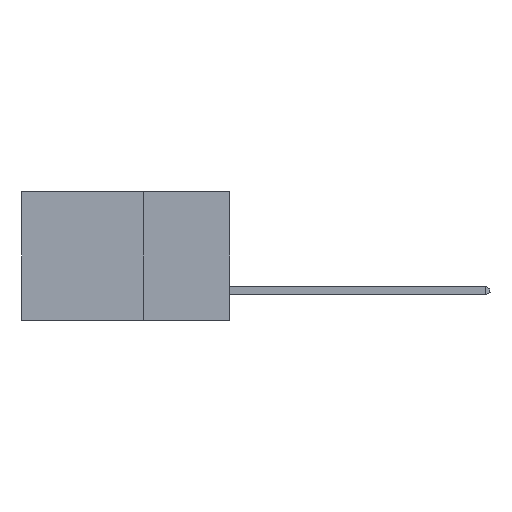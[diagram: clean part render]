
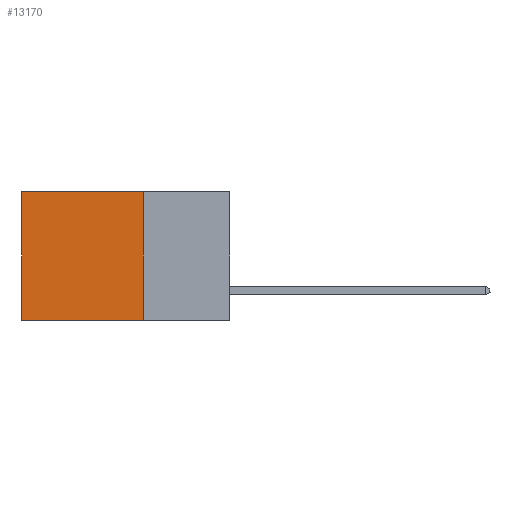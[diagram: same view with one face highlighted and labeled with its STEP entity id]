
A CAD part, left-side view. The second image highlights one B-rep face of the part: STEP entity #13170.
In plain terms, the highlighted planar face has unit normal (-1, 0, 0).
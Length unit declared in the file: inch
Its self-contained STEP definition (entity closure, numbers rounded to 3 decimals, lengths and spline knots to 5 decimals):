
#212 = LINE ( 'NONE', #4248, #2225 ) ;
#361 = DIRECTION ( 'NONE',  ( 1., 0., 0. ) ) ;
#650 = LINE ( 'NONE', #12073, #17280 ) ;
#757 = LINE ( 'NONE', #10620, #15401 ) ;
#853 = VERTEX_POINT ( 'NONE', #14147 ) ;
#2225 = VECTOR ( 'NONE', #9693, 39.37008 ) ;
#2422 = EDGE_CURVE ( 'NONE', #6569, #853, #212, .T. ) ;
#2776 = EDGE_CURVE ( 'NONE', #10429, #11926, #650, .T. ) ;
#3366 = ORIENTED_EDGE ( 'NONE', *, *, #5352, .T. ) ;
#4248 = CARTESIAN_POINT ( 'NONE',  ( 0.298, 0.25, 0. ) ) ;
#4781 = PLANE ( 'NONE',  #13228 ) ;
#5352 = EDGE_CURVE ( 'NONE', #853, #11926, #757, .T. ) ;
#5887 = DIRECTION ( 'NONE',  ( 0., 0., -1. ) ) ;
#6569 = VERTEX_POINT ( 'NONE', #12617 ) ;
#7108 = FACE_OUTER_BOUND ( 'NONE', #10901, .T. ) ;
#7660 = CARTESIAN_POINT ( 'NONE',  ( 0.298, 0.25, -0.37 ) ) ;
#9371 = DIRECTION ( 'NONE',  ( 0., 1., 0. ) ) ;
#9376 = ORIENTED_EDGE ( 'NONE', *, *, #2776, .F. ) ;
#9652 = ORIENTED_EDGE ( 'NONE', *, *, #2422, .T. ) ;
#9693 = DIRECTION ( 'NONE',  ( 0., 1., 0. ) ) ;
#10429 = VERTEX_POINT ( 'NONE', #7660 ) ;
#10620 = CARTESIAN_POINT ( 'NONE',  ( 0.298, 0.6, 0. ) ) ;
#10673 = VECTOR ( 'NONE', #11463, 39.37008 ) ;
#10838 = CARTESIAN_POINT ( 'NONE',  ( 0.298, 0.6, -0.37 ) ) ;
#10901 = EDGE_LOOP ( 'NONE', ( #3366, #9376, #17614, #9652 ) ) ;
#11463 = DIRECTION ( 'NONE',  ( 0., 0., -1. ) ) ;
#11926 = VERTEX_POINT ( 'NONE', #10838 ) ;
#12073 = CARTESIAN_POINT ( 'NONE',  ( 0.298, 0.25, -0.37 ) ) ;
#12617 = CARTESIAN_POINT ( 'NONE',  ( 0.298, 0.25, 0. ) ) ;
#12894 = EDGE_CURVE ( 'NONE', #6569, #10429, #17350, .T. ) ;
#13100 = CARTESIAN_POINT ( 'NONE',  ( 0.298, 0.25, 0. ) ) ;
#13170 = ADVANCED_FACE ( 'NONE', ( #7108 ), #4781, .F. ) ;
#13228 = AXIS2_PLACEMENT_3D ( 'NONE', #13100, #361, #5887 ) ;
#14147 = CARTESIAN_POINT ( 'NONE',  ( 0.298, 0.6, 0. ) ) ;
#15401 = VECTOR ( 'NONE', #17650, 39.37008 ) ;
#15775 = CARTESIAN_POINT ( 'NONE',  ( 0.298, 0.25, 0. ) ) ;
#17280 = VECTOR ( 'NONE', #9371, 39.37008 ) ;
#17350 = LINE ( 'NONE', #15775, #10673 ) ;
#17614 = ORIENTED_EDGE ( 'NONE', *, *, #12894, .F. ) ;
#17650 = DIRECTION ( 'NONE',  ( 0., 0., -1. ) ) ;
